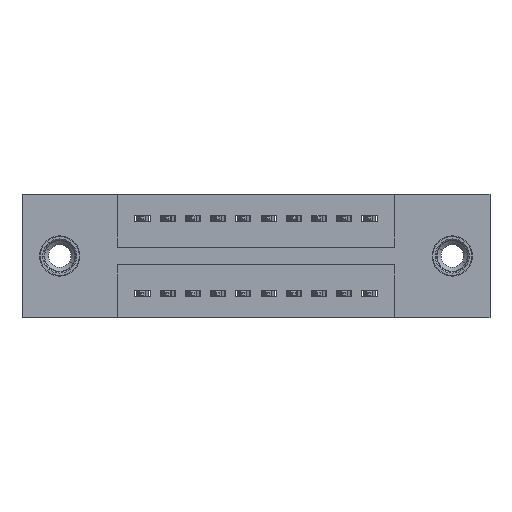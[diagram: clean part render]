
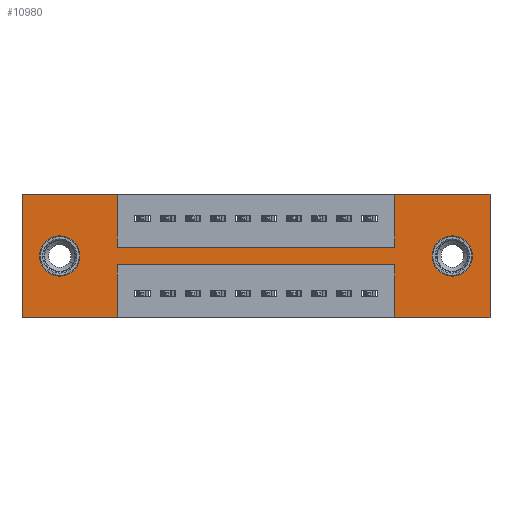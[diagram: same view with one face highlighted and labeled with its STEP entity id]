
A CAD part, front view. The second image highlights one B-rep face of the part: STEP entity #10980.
In plain terms, the highlighted planar face has unit normal (0, -1, 0).
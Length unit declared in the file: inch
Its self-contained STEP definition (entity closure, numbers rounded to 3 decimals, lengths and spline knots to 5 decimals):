
#43 = CARTESIAN_POINT ( 'NONE',  ( 0.1495, 0., -0.245 ) ) ;
#72 = CARTESIAN_POINT ( 'NONE',  ( 1.4775, 0., -0.28 ) ) ;
#181 = CARTESIAN_POINT ( 'NONE',  ( 0.3775, 0., -0.21 ) ) ;
#249 = LINE ( 'NONE', #7489, #4184 ) ;
#289 = CARTESIAN_POINT ( 'NONE',  ( 1.7055, 0., -0.245 ) ) ;
#349 = ORIENTED_EDGE ( 'NONE', *, *, #3943, .F. ) ;
#443 = VECTOR ( 'NONE', #5912, 39.37008 ) ;
#491 = CIRCLE ( 'NONE', #2852, 0.08 ) ;
#502 = LINE ( 'NONE', #11229, #4463 ) ;
#509 = ORIENTED_EDGE ( 'NONE', *, *, #8694, .F. ) ;
#530 = CIRCLE ( 'NONE', #11067, 0.08 ) ;
#555 = DIRECTION ( 'NONE',  ( 0., 1., 0. ) ) ;
#710 = EDGE_CURVE ( 'NONE', #3892, #2735, #9089, .T. ) ;
#933 = PLANE ( 'NONE',  #7797 ) ;
#1097 = CARTESIAN_POINT ( 'NONE',  ( 0., 0., 0. ) ) ;
#1098 = ORIENTED_EDGE ( 'NONE', *, *, #11128, .F. ) ;
#1178 = DIRECTION ( 'NONE',  ( 0., 0., -1. ) ) ;
#1192 = ORIENTED_EDGE ( 'NONE', *, *, #6488, .F. ) ;
#1306 = DIRECTION ( 'NONE',  ( -1., 0., 0. ) ) ;
#1321 = VERTEX_POINT ( 'NONE', #2222 ) ;
#1473 = VERTEX_POINT ( 'NONE', #9506 ) ;
#1483 = ORIENTED_EDGE ( 'NONE', *, *, #3020, .T. ) ;
#1607 = VERTEX_POINT ( 'NONE', #8056 ) ;
#1756 = DIRECTION ( 'NONE',  ( 0., 0., -1. ) ) ;
#1768 = CARTESIAN_POINT ( 'NONE',  ( 0.3775, 0., 0. ) ) ;
#1808 = LINE ( 'NONE', #10375, #8928 ) ;
#1809 = DIRECTION ( 'NONE',  ( 0., 1., 0. ) ) ;
#2120 = DIRECTION ( 'NONE',  ( 0., 1., 0. ) ) ;
#2222 = CARTESIAN_POINT ( 'NONE',  ( 1.4775, 0., 0. ) ) ;
#2290 = VERTEX_POINT ( 'NONE', #8151 ) ;
#2422 = VECTOR ( 'NONE', #11749, 39.37008 ) ;
#2472 = DIRECTION ( 'NONE',  ( 0., 0., -1. ) ) ;
#2564 = EDGE_CURVE ( 'NONE', #2290, #1607, #1808, .T. ) ;
#2597 = DIRECTION ( 'NONE',  ( 0., 1., 0. ) ) ;
#2612 = ORIENTED_EDGE ( 'NONE', *, *, #2564, .F. ) ;
#2628 = ORIENTED_EDGE ( 'NONE', *, *, #7911, .F. ) ;
#2735 = VERTEX_POINT ( 'NONE', #7553 ) ;
#2806 = FACE_OUTER_BOUND ( 'NONE', #11219, .T. ) ;
#2852 = AXIS2_PLACEMENT_3D ( 'NONE', #289, #2120, #1178 ) ;
#2870 = VERTEX_POINT ( 'NONE', #9107 ) ;
#2912 = VERTEX_POINT ( 'NONE', #4588 ) ;
#2938 = VECTOR ( 'NONE', #8846, 39.37008 ) ;
#2939 = CARTESIAN_POINT ( 'NONE',  ( 0.3775, 0., -0.21 ) ) ;
#3020 = EDGE_CURVE ( 'NONE', #3691, #1473, #530, .T. ) ;
#3049 = DIRECTION ( 'NONE',  ( -1., 0., 0. ) ) ;
#3199 = CARTESIAN_POINT ( 'NONE',  ( 0.3775, 0., -0.28 ) ) ;
#3232 = CIRCLE ( 'NONE', #8913, 0.08 ) ;
#3318 = EDGE_CURVE ( 'NONE', #4615, #9464, #8341, .T. ) ;
#3336 = ORIENTED_EDGE ( 'NONE', *, *, #11242, .F. ) ;
#3651 = EDGE_CURVE ( 'NONE', #2912, #9368, #10939, .T. ) ;
#3691 = VERTEX_POINT ( 'NONE', #5728 ) ;
#3840 = CARTESIAN_POINT ( 'NONE',  ( 1.4775, 0., -0.21 ) ) ;
#3892 = VERTEX_POINT ( 'NONE', #11268 ) ;
#3900 = ORIENTED_EDGE ( 'NONE', *, *, #4429, .T. ) ;
#3914 = ORIENTED_EDGE ( 'NONE', *, *, #8112, .F. ) ;
#3943 = EDGE_CURVE ( 'NONE', #2870, #9498, #502, .T. ) ;
#4184 = VECTOR ( 'NONE', #3049, 39.37008 ) ;
#4207 = FACE_BOUND ( 'NONE', #8005, .T. ) ;
#4424 = CARTESIAN_POINT ( 'NONE',  ( 0.1495, 0., -0.245 ) ) ;
#4429 = EDGE_CURVE ( 'NONE', #2735, #3892, #491, .T. ) ;
#4437 = CARTESIAN_POINT ( 'NONE',  ( 0., 0., -0.49 ) ) ;
#4463 = VECTOR ( 'NONE', #7660, 39.37008 ) ;
#4588 = CARTESIAN_POINT ( 'NONE',  ( 1.4775, 0., -0.49 ) ) ;
#4615 = VERTEX_POINT ( 'NONE', #1768 ) ;
#4775 = ORIENTED_EDGE ( 'NONE', *, *, #11554, .F. ) ;
#4828 = CARTESIAN_POINT ( 'NONE',  ( 0., 0., 0. ) ) ;
#5095 = DIRECTION ( 'NONE',  ( 0., 0., -1. ) ) ;
#5226 = CARTESIAN_POINT ( 'NONE',  ( 1.855, 0., -0.49 ) ) ;
#5254 = AXIS2_PLACEMENT_3D ( 'NONE', #11477, #555, #5095 ) ;
#5314 = ORIENTED_EDGE ( 'NONE', *, *, #11540, .F. ) ;
#5432 = ORIENTED_EDGE ( 'NONE', *, *, #10510, .T. ) ;
#5462 = DIRECTION ( 'NONE',  ( 0., 0., 1. ) ) ;
#5716 = CARTESIAN_POINT ( 'NONE',  ( 1.4775, 0., -0.21 ) ) ;
#5728 = CARTESIAN_POINT ( 'NONE',  ( 0.1495, 0., -0.165 ) ) ;
#5782 = DIRECTION ( 'NONE',  ( 1., 0., 0. ) ) ;
#5874 = CARTESIAN_POINT ( 'NONE',  ( 0., 0., 0. ) ) ;
#5912 = DIRECTION ( 'NONE',  ( 1., 0., 0. ) ) ;
#5998 = EDGE_LOOP ( 'NONE', ( #1483, #5432 ) ) ;
#6037 = LINE ( 'NONE', #6111, #2938 ) ;
#6041 = VERTEX_POINT ( 'NONE', #10459 ) ;
#6111 = CARTESIAN_POINT ( 'NONE',  ( 1.855, 0., 0. ) ) ;
#6231 = VECTOR ( 'NONE', #10345, 39.37008 ) ;
#6360 = LINE ( 'NONE', #7189, #2422 ) ;
#6407 = VECTOR ( 'NONE', #5782, 39.37008 ) ;
#6488 = EDGE_CURVE ( 'NONE', #7055, #1321, #9975, .T. ) ;
#6507 = DIRECTION ( 'NONE',  ( 0., 0., 1. ) ) ;
#7039 = VECTOR ( 'NONE', #10963, 39.37008 ) ;
#7055 = VERTEX_POINT ( 'NONE', #5716 ) ;
#7100 = ORIENTED_EDGE ( 'NONE', *, *, #3318, .F. ) ;
#7134 = CARTESIAN_POINT ( 'NONE',  ( 1.4775, 0., -0.28 ) ) ;
#7189 = CARTESIAN_POINT ( 'NONE',  ( 0., 0., -0.49 ) ) ;
#7283 = DIRECTION ( 'NONE',  ( 0., -1., 0. ) ) ;
#7370 = DIRECTION ( 'NONE',  ( 1., 0., 0. ) ) ;
#7489 = CARTESIAN_POINT ( 'NONE',  ( 0., 0., -0.49 ) ) ;
#7553 = CARTESIAN_POINT ( 'NONE',  ( 1.7055, 0., -0.165 ) ) ;
#7660 = DIRECTION ( 'NONE',  ( 0., 0., 1. ) ) ;
#7797 = AXIS2_PLACEMENT_3D ( 'NONE', #4437, #7283, #1756 ) ;
#7911 = EDGE_CURVE ( 'NONE', #1607, #2870, #249, .T. ) ;
#8005 = EDGE_LOOP ( 'NONE', ( #3900, #9726 ) ) ;
#8048 = VECTOR ( 'NONE', #1306, 39.37008 ) ;
#8056 = CARTESIAN_POINT ( 'NONE',  ( 0.3775, 0., -0.49 ) ) ;
#8112 = EDGE_CURVE ( 'NONE', #9368, #2290, #10495, .T. ) ;
#8151 = CARTESIAN_POINT ( 'NONE',  ( 0.3775, 0., -0.28 ) ) ;
#8341 = LINE ( 'NONE', #8692, #11241 ) ;
#8408 = LINE ( 'NONE', #4828, #6407 ) ;
#8531 = DIRECTION ( 'NONE',  ( 0., 0., -1. ) ) ;
#8692 = CARTESIAN_POINT ( 'NONE',  ( 0.3775, 0., -0.21 ) ) ;
#8694 = EDGE_CURVE ( 'NONE', #1321, #6041, #8408, .T. ) ;
#8846 = DIRECTION ( 'NONE',  ( 0., 0., -1. ) ) ;
#8913 = AXIS2_PLACEMENT_3D ( 'NONE', #4424, #2597, #5462 ) ;
#8928 = VECTOR ( 'NONE', #8531, 39.37008 ) ;
#9089 = CIRCLE ( 'NONE', #5254, 0.08 ) ;
#9107 = CARTESIAN_POINT ( 'NONE',  ( 0., 0., -0.49 ) ) ;
#9121 = LINE ( 'NONE', #5874, #443 ) ;
#9368 = VERTEX_POINT ( 'NONE', #72 ) ;
#9464 = VERTEX_POINT ( 'NONE', #2939 ) ;
#9498 = VERTEX_POINT ( 'NONE', #1097 ) ;
#9506 = CARTESIAN_POINT ( 'NONE',  ( 0.1495, 0., -0.325 ) ) ;
#9726 = ORIENTED_EDGE ( 'NONE', *, *, #710, .T. ) ;
#9824 = LINE ( 'NONE', #181, #10532 ) ;
#9975 = LINE ( 'NONE', #3840, #6231 ) ;
#10334 = ORIENTED_EDGE ( 'NONE', *, *, #3651, .F. ) ;
#10345 = DIRECTION ( 'NONE',  ( 0., 0., 1. ) ) ;
#10375 = CARTESIAN_POINT ( 'NONE',  ( 0.3775, 0., -0.28 ) ) ;
#10459 = CARTESIAN_POINT ( 'NONE',  ( 1.855, 0., 0. ) ) ;
#10495 = LINE ( 'NONE', #3199, #8048 ) ;
#10510 = EDGE_CURVE ( 'NONE', #1473, #3691, #3232, .T. ) ;
#10532 = VECTOR ( 'NONE', #7370, 39.37008 ) ;
#10916 = VERTEX_POINT ( 'NONE', #5226 ) ;
#10939 = LINE ( 'NONE', #7134, #7039 ) ;
#10963 = DIRECTION ( 'NONE',  ( 0., 0., 1. ) ) ;
#10980 = ADVANCED_FACE ( 'NONE', ( #4207, #11525, #2806 ), #933, .T. ) ;
#11067 = AXIS2_PLACEMENT_3D ( 'NONE', #43, #1809, #6507 ) ;
#11128 = EDGE_CURVE ( 'NONE', #9464, #7055, #9824, .T. ) ;
#11219 = EDGE_LOOP ( 'NONE', ( #1192, #1098, #7100, #3336, #349, #2628, #2612, #3914, #10334, #4775, #5314, #509 ) ) ;
#11229 = CARTESIAN_POINT ( 'NONE',  ( 0., 0., 0. ) ) ;
#11241 = VECTOR ( 'NONE', #2472, 39.37008 ) ;
#11242 = EDGE_CURVE ( 'NONE', #9498, #4615, #9121, .T. ) ;
#11268 = CARTESIAN_POINT ( 'NONE',  ( 1.7055, 0., -0.325 ) ) ;
#11477 = CARTESIAN_POINT ( 'NONE',  ( 1.7055, 0., -0.245 ) ) ;
#11525 = FACE_BOUND ( 'NONE', #5998, .T. ) ;
#11540 = EDGE_CURVE ( 'NONE', #6041, #10916, #6037, .T. ) ;
#11554 = EDGE_CURVE ( 'NONE', #10916, #2912, #6360, .T. ) ;
#11749 = DIRECTION ( 'NONE',  ( -1., 0., 0. ) ) ;
